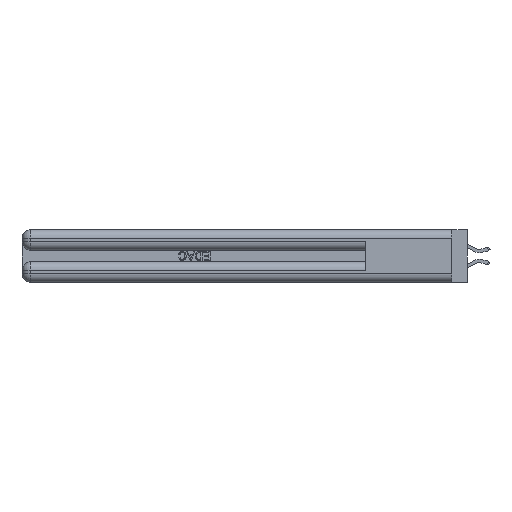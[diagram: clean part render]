
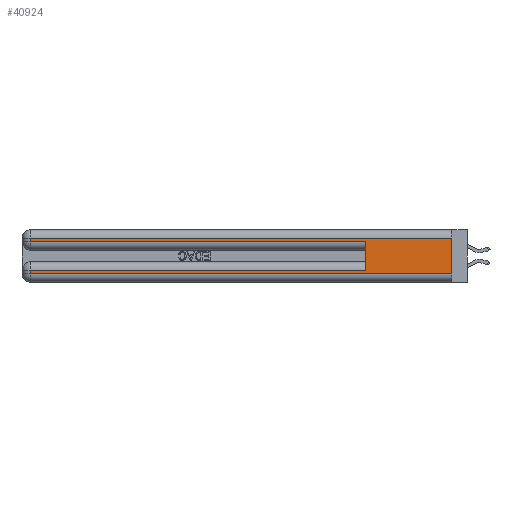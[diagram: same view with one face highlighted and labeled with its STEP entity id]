
A CAD part, left-side view. The second image highlights one B-rep face of the part: STEP entity #40924.
In plain terms, the highlighted planar face has unit normal (-1, 0, 0).
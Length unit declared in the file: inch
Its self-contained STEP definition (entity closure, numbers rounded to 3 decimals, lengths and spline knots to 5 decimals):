
#1826 = VERTEX_POINT ( 'NONE', #37428 ) ;
#2834 = CARTESIAN_POINT ( 'NONE',  ( 0., 2.94, 0.37 ) ) ;
#3053 = ORIENTED_EDGE ( 'NONE', *, *, #25494, .T. ) ;
#3197 = ORIENTED_EDGE ( 'NONE', *, *, #40714, .T. ) ;
#3456 = EDGE_CURVE ( 'NONE', #1826, #16979, #31209, .T. ) ;
#3897 = CARTESIAN_POINT ( 'NONE',  ( 0., 0., 0.37 ) ) ;
#4232 = VERTEX_POINT ( 'NONE', #42291 ) ;
#6109 = VECTOR ( 'NONE', #37133, 39.37008 ) ;
#6589 = LINE ( 'NONE', #16049, #42962 ) ;
#7165 = CARTESIAN_POINT ( 'NONE',  ( 0., 2.94, 0.37 ) ) ;
#7479 = DIRECTION ( 'NONE',  ( 0., 0., -1. ) ) ;
#8210 = LINE ( 'NONE', #22146, #44568 ) ;
#8666 = ORIENTED_EDGE ( 'NONE', *, *, #20144, .T. ) ;
#9857 = VERTEX_POINT ( 'NONE', #44789 ) ;
#11167 = VECTOR ( 'NONE', #20379, 39.37008 ) ;
#12096 = EDGE_CURVE ( 'NONE', #4232, #37842, #14143, .T. ) ;
#14143 = LINE ( 'NONE', #37127, #32930 ) ;
#14456 = VECTOR ( 'NONE', #28585, 39.37008 ) ;
#14697 = ORIENTED_EDGE ( 'NONE', *, *, #31701, .T. ) ;
#16049 = CARTESIAN_POINT ( 'NONE',  ( 0., 0., 0.085 ) ) ;
#16284 = CARTESIAN_POINT ( 'NONE',  ( 0., 2.94, 0.31 ) ) ;
#16979 = VERTEX_POINT ( 'NONE', #24466 ) ;
#16992 = CARTESIAN_POINT ( 'NONE',  ( 0., 0., 0.06 ) ) ;
#18059 = PLANE ( 'NONE',  #21108 ) ;
#18203 = ORIENTED_EDGE ( 'NONE', *, *, #3456, .T. ) ;
#19573 = DIRECTION ( 'NONE',  ( 0., 0., 1. ) ) ;
#20028 = FACE_OUTER_BOUND ( 'NONE', #43608, .T. ) ;
#20084 = ORIENTED_EDGE ( 'NONE', *, *, #41062, .F. ) ;
#20144 = EDGE_CURVE ( 'NONE', #4232, #1826, #6589, .T. ) ;
#20379 = DIRECTION ( 'NONE',  ( 0., -1., 0. ) ) ;
#21108 = AXIS2_PLACEMENT_3D ( 'NONE', #3897, #28750, #7479 ) ;
#22146 = CARTESIAN_POINT ( 'NONE',  ( 0., 0., 0.285 ) ) ;
#23182 = DIRECTION ( 'NONE',  ( 0., 1., 0. ) ) ;
#24466 = CARTESIAN_POINT ( 'NONE',  ( 0., 2.94, 0.06 ) ) ;
#25236 = CARTESIAN_POINT ( 'NONE',  ( 0., 0., 0.31 ) ) ;
#25494 = EDGE_CURVE ( 'NONE', #34000, #29617, #33238, .T. ) ;
#25858 = ORIENTED_EDGE ( 'NONE', *, *, #12096, .F. ) ;
#26354 = EDGE_CURVE ( 'NONE', #29617, #37842, #8210, .T. ) ;
#26537 = CARTESIAN_POINT ( 'NONE',  ( 0., 0., 0.37 ) ) ;
#27669 = LINE ( 'NONE', #44856, #35909 ) ;
#27697 = DIRECTION ( 'NONE',  ( 0., 0., -1. ) ) ;
#28585 = DIRECTION ( 'NONE',  ( 0., 0., -1. ) ) ;
#28718 = CARTESIAN_POINT ( 'NONE',  ( 0., 2.94, 0.285 ) ) ;
#28750 = DIRECTION ( 'NONE',  ( 1., 0., 0. ) ) ;
#29269 = DIRECTION ( 'NONE',  ( 0., -1., 0. ) ) ;
#29617 = VERTEX_POINT ( 'NONE', #28718 ) ;
#30822 = CARTESIAN_POINT ( 'NONE',  ( 0., 0.6, 0.285 ) ) ;
#30851 = ORIENTED_EDGE ( 'NONE', *, *, #26354, .T. ) ;
#31209 = LINE ( 'NONE', #2834, #41571 ) ;
#31701 = EDGE_CURVE ( 'NONE', #38126, #34000, #27669, .T. ) ;
#32930 = VECTOR ( 'NONE', #19573, 39.37008 ) ;
#33238 = LINE ( 'NONE', #7165, #14456 ) ;
#34000 = VERTEX_POINT ( 'NONE', #16284 ) ;
#35909 = VECTOR ( 'NONE', #41386, 39.37008 ) ;
#37127 = CARTESIAN_POINT ( 'NONE',  ( 0., 0.6, 0.145 ) ) ;
#37133 = DIRECTION ( 'NONE',  ( 0., 0., -1. ) ) ;
#37428 = CARTESIAN_POINT ( 'NONE',  ( 0., 2.94, 0.085 ) ) ;
#37842 = VERTEX_POINT ( 'NONE', #30822 ) ;
#38126 = VERTEX_POINT ( 'NONE', #25236 ) ;
#38225 = LINE ( 'NONE', #16992, #11167 ) ;
#40714 = EDGE_CURVE ( 'NONE', #16979, #9857, #38225, .T. ) ;
#40924 = ADVANCED_FACE ( 'NONE', ( #20028 ), #18059, .F. ) ;
#41062 = EDGE_CURVE ( 'NONE', #38126, #9857, #44678, .T. ) ;
#41386 = DIRECTION ( 'NONE',  ( 0., 1., 0. ) ) ;
#41571 = VECTOR ( 'NONE', #27697, 39.37008 ) ;
#42291 = CARTESIAN_POINT ( 'NONE',  ( 0., 0.6, 0.085 ) ) ;
#42962 = VECTOR ( 'NONE', #23182, 39.37008 ) ;
#43608 = EDGE_LOOP ( 'NONE', ( #20084, #14697, #3053, #30851, #25858, #8666, #18203, #3197 ) ) ;
#44568 = VECTOR ( 'NONE', #29269, 39.37008 ) ;
#44678 = LINE ( 'NONE', #26537, #6109 ) ;
#44789 = CARTESIAN_POINT ( 'NONE',  ( 0., 0., 0.06 ) ) ;
#44856 = CARTESIAN_POINT ( 'NONE',  ( 0., 0., 0.31 ) ) ;
